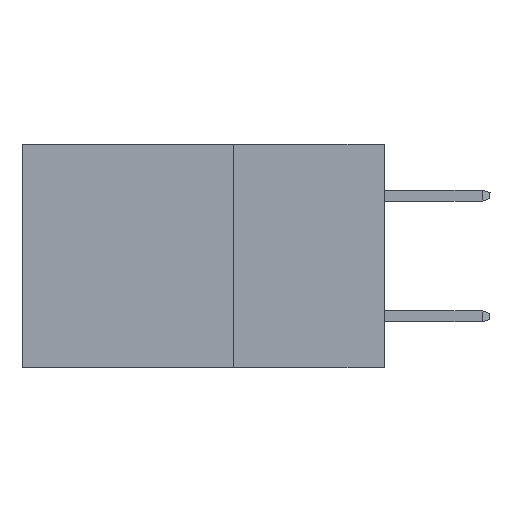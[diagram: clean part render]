
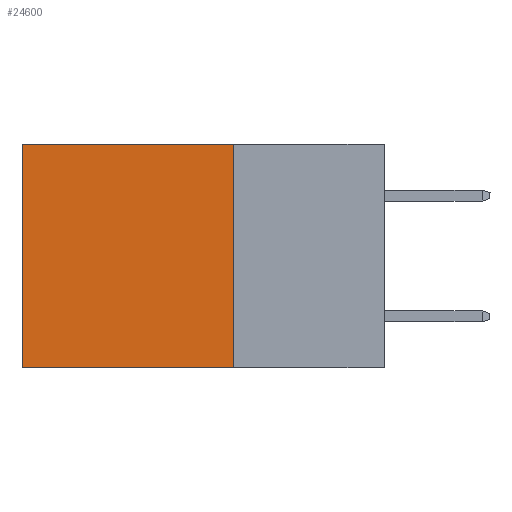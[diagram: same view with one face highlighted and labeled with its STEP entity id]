
A CAD part, left-side view. The second image highlights one B-rep face of the part: STEP entity #24600.
In plain terms, the highlighted planar face has unit normal (-1, 0, 0).
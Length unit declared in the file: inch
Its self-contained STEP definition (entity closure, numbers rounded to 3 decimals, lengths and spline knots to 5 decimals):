
#1056 = CARTESIAN_POINT ( 'NONE',  ( 0.298, 0.25, 0. ) ) ;
#3274 = ORIENTED_EDGE ( 'NONE', *, *, #20671, .T. ) ;
#3507 = LINE ( 'NONE', #13758, #15641 ) ;
#4903 = VERTEX_POINT ( 'NONE', #7300 ) ;
#5432 = FACE_OUTER_BOUND ( 'NONE', #18483, .T. ) ;
#5629 = ORIENTED_EDGE ( 'NONE', *, *, #17698, .T. ) ;
#6055 = CARTESIAN_POINT ( 'NONE',  ( 0.298, 0.25, 0. ) ) ;
#6807 = CARTESIAN_POINT ( 'NONE',  ( 0.298, 0.6, -0.37 ) ) ;
#7213 = ORIENTED_EDGE ( 'NONE', *, *, #10343, .F. ) ;
#7300 = CARTESIAN_POINT ( 'NONE',  ( 0.298, 0.6, 0. ) ) ;
#8071 = LINE ( 'NONE', #13157, #18477 ) ;
#8287 = EDGE_CURVE ( 'NONE', #12806, #25245, #27999, .T. ) ;
#8979 = AXIS2_PLACEMENT_3D ( 'NONE', #12829, #15179, #19835 ) ;
#10327 = VECTOR ( 'NONE', #14838, 39.37008 ) ;
#10343 = EDGE_CURVE ( 'NONE', #10616, #12806, #21710, .T. ) ;
#10616 = VERTEX_POINT ( 'NONE', #6055 ) ;
#12165 = DIRECTION ( 'NONE',  ( 0., 0., -1. ) ) ;
#12806 = VERTEX_POINT ( 'NONE', #20969 ) ;
#12829 = CARTESIAN_POINT ( 'NONE',  ( 0.298, 0.25, 0. ) ) ;
#13157 = CARTESIAN_POINT ( 'NONE',  ( 0.298, 0.25, 0. ) ) ;
#13758 = CARTESIAN_POINT ( 'NONE',  ( 0.298, 0.6, 0. ) ) ;
#14838 = DIRECTION ( 'NONE',  ( 0., 1., 0. ) ) ;
#15179 = DIRECTION ( 'NONE',  ( 1., 0., 0. ) ) ;
#15641 = VECTOR ( 'NONE', #16277, 39.37008 ) ;
#16277 = DIRECTION ( 'NONE',  ( 0., 0., -1. ) ) ;
#17698 = EDGE_CURVE ( 'NONE', #4903, #25245, #3507, .T. ) ;
#18477 = VECTOR ( 'NONE', #21600, 39.37008 ) ;
#18483 = EDGE_LOOP ( 'NONE', ( #5629, #19739, #7213, #3274 ) ) ;
#19739 = ORIENTED_EDGE ( 'NONE', *, *, #8287, .F. ) ;
#19835 = DIRECTION ( 'NONE',  ( 0., 0., -1. ) ) ;
#20671 = EDGE_CURVE ( 'NONE', #10616, #4903, #8071, .T. ) ;
#20969 = CARTESIAN_POINT ( 'NONE',  ( 0.298, 0.25, -0.37 ) ) ;
#21600 = DIRECTION ( 'NONE',  ( 0., 1., 0. ) ) ;
#21710 = LINE ( 'NONE', #1056, #28632 ) ;
#23875 = CARTESIAN_POINT ( 'NONE',  ( 0.298, 0.25, -0.37 ) ) ;
#24600 = ADVANCED_FACE ( 'NONE', ( #5432 ), #26233, .F. ) ;
#25245 = VERTEX_POINT ( 'NONE', #6807 ) ;
#26233 = PLANE ( 'NONE',  #8979 ) ;
#27999 = LINE ( 'NONE', #23875, #10327 ) ;
#28632 = VECTOR ( 'NONE', #12165, 39.37008 ) ;
